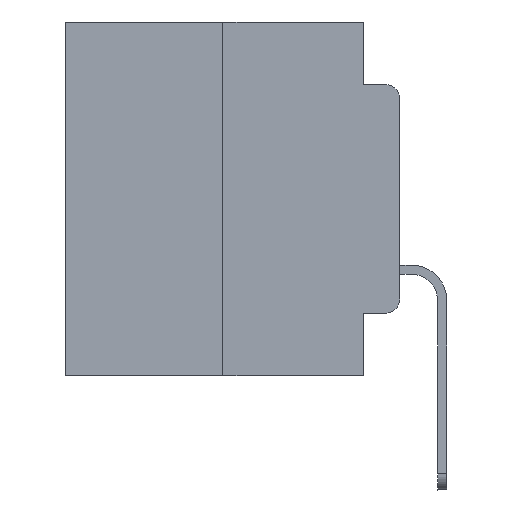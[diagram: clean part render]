
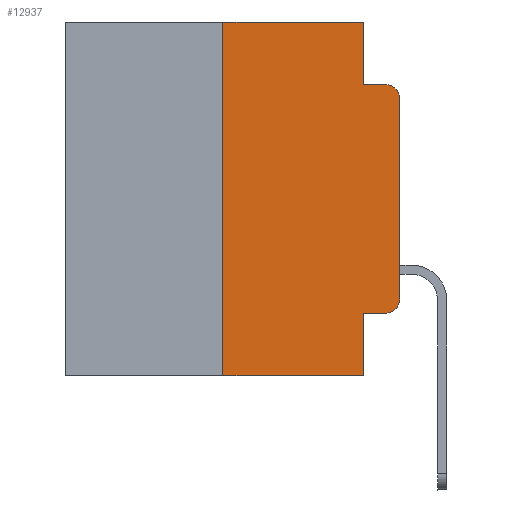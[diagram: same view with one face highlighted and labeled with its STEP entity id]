
A CAD part, left-side view. The second image highlights one B-rep face of the part: STEP entity #12937.
In plain terms, the highlighted planar face has unit normal (-1, 0, 0).
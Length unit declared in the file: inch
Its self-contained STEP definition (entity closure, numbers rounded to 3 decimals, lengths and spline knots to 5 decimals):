
#37 = VERTEX_POINT ( 'NONE', #889 ) ;
#81 = VERTEX_POINT ( 'NONE', #19235 ) ;
#333 = CIRCLE ( 'NONE', #19861, 0.02 ) ;
#505 = AXIS2_PLACEMENT_3D ( 'NONE', #17431, #948, #13442 ) ;
#548 = ORIENTED_EDGE ( 'NONE', *, *, #4891, .T. ) ;
#727 = LINE ( 'NONE', #10863, #883 ) ;
#883 = VECTOR ( 'NONE', #7252, 39.37008 ) ;
#889 = CARTESIAN_POINT ( 'NONE',  ( 0., 0.25, -0.5 ) ) ;
#948 = DIRECTION ( 'NONE',  ( 1., 0., 0. ) ) ;
#1350 = CARTESIAN_POINT ( 'NONE',  ( 0., 0.051, -0.4115 ) ) ;
#1603 = VERTEX_POINT ( 'NONE', #5656 ) ;
#1618 = VERTEX_POINT ( 'NONE', #5376 ) ;
#2019 = VECTOR ( 'NONE', #16478, 39.37008 ) ;
#3756 = VERTEX_POINT ( 'NONE', #25233 ) ;
#3914 = EDGE_LOOP ( 'NONE', ( #16381, #23567, #5466, #25305, #15604, #6276, #548, #19834, #11335, #19244 ) ) ;
#4144 = EDGE_CURVE ( 'NONE', #81, #17900, #727, .T. ) ;
#4157 = CARTESIAN_POINT ( 'NONE',  ( 0., 0.051, 0. ) ) ;
#4180 = VERTEX_POINT ( 'NONE', #17103 ) ;
#4891 = EDGE_CURVE ( 'NONE', #37, #17900, #12891, .T. ) ;
#5034 = CARTESIAN_POINT ( 'NONE',  ( 0., 0.02, -0.1085 ) ) ;
#5376 = CARTESIAN_POINT ( 'NONE',  ( 0., 0.02, -0.0885 ) ) ;
#5466 = ORIENTED_EDGE ( 'NONE', *, *, #22309, .F. ) ;
#5656 = CARTESIAN_POINT ( 'NONE',  ( 0., 0., -0.1085 ) ) ;
#6098 = LINE ( 'NONE', #6337, #12428 ) ;
#6172 = LINE ( 'NONE', #4157, #25601 ) ;
#6267 = CARTESIAN_POINT ( 'NONE',  ( 0., 0.051, 0. ) ) ;
#6276 = ORIENTED_EDGE ( 'NONE', *, *, #20710, .F. ) ;
#6282 = AXIS2_PLACEMENT_3D ( 'NONE', #9366, #13472, #17469 ) ;
#6337 = CARTESIAN_POINT ( 'NONE',  ( 0., 0., 0. ) ) ;
#6486 = CARTESIAN_POINT ( 'NONE',  ( 0., 0., -0.3915 ) ) ;
#7252 = DIRECTION ( 'NONE',  ( 0., 0., -1. ) ) ;
#7475 = CARTESIAN_POINT ( 'NONE',  ( 0., 0.051, -0.5 ) ) ;
#8793 = CARTESIAN_POINT ( 'NONE',  ( 0., 0.051, -0.0885 ) ) ;
#8844 = CIRCLE ( 'NONE', #6282, 0.02 ) ;
#8915 = DIRECTION ( 'NONE',  ( 0., 0., -1. ) ) ;
#9297 = DIRECTION ( 'NONE',  ( 0., -1., 0. ) ) ;
#9366 = CARTESIAN_POINT ( 'NONE',  ( 0., 0.02, -0.3915 ) ) ;
#9746 = LINE ( 'NONE', #1350, #24771 ) ;
#10002 = VERTEX_POINT ( 'NONE', #8793 ) ;
#10120 = CARTESIAN_POINT ( 'NONE',  ( 0., 0.473, 0. ) ) ;
#10453 = VERTEX_POINT ( 'NONE', #6486 ) ;
#10511 = CARTESIAN_POINT ( 'NONE',  ( 0., 0.051, -0.0885 ) ) ;
#10863 = CARTESIAN_POINT ( 'NONE',  ( 0., 0.051, 0. ) ) ;
#11335 = ORIENTED_EDGE ( 'NONE', *, *, #19084, .T. ) ;
#12288 = DIRECTION ( 'NONE',  ( 0., 0., -1. ) ) ;
#12428 = VECTOR ( 'NONE', #20310, 39.37008 ) ;
#12651 = CARTESIAN_POINT ( 'NONE',  ( 0., 0.25, 0. ) ) ;
#12891 = LINE ( 'NONE', #16866, #25067 ) ;
#12937 = ADVANCED_FACE ( 'NONE', ( #19157 ), #17044, .F. ) ;
#13017 = DIRECTION ( 'NONE',  ( 0., -1., 0. ) ) ;
#13349 = EDGE_CURVE ( 'NONE', #3756, #19310, #14244, .T. ) ;
#13442 = DIRECTION ( 'NONE',  ( 0., 0., -1. ) ) ;
#13472 = DIRECTION ( 'NONE',  ( -1., 0., 0. ) ) ;
#13610 = EDGE_CURVE ( 'NONE', #10453, #1603, #6098, .T. ) ;
#14244 = LINE ( 'NONE', #10120, #24319 ) ;
#14882 = DIRECTION ( 'NONE',  ( -1., 0., 0. ) ) ;
#15604 = ORIENTED_EDGE ( 'NONE', *, *, #13349, .F. ) ;
#16381 = ORIENTED_EDGE ( 'NONE', *, *, #13610, .T. ) ;
#16478 = DIRECTION ( 'NONE',  ( 0., -1., 0. ) ) ;
#16866 = CARTESIAN_POINT ( 'NONE',  ( 0., 0.473, -0.5 ) ) ;
#17039 = LINE ( 'NONE', #12651, #23143 ) ;
#17044 = PLANE ( 'NONE',  #505 ) ;
#17103 = CARTESIAN_POINT ( 'NONE',  ( 0., 0.02, -0.4115 ) ) ;
#17431 = CARTESIAN_POINT ( 'NONE',  ( 0., 0.473, 0. ) ) ;
#17469 = DIRECTION ( 'NONE',  ( 0., 0., -1. ) ) ;
#17725 = LINE ( 'NONE', #10511, #2019 ) ;
#17900 = VERTEX_POINT ( 'NONE', #7475 ) ;
#18891 = DIRECTION ( 'NONE',  ( 0., 0., 1. ) ) ;
#18921 = EDGE_CURVE ( 'NONE', #19310, #10002, #6172, .T. ) ;
#19084 = EDGE_CURVE ( 'NONE', #81, #4180, #9746, .T. ) ;
#19157 = FACE_OUTER_BOUND ( 'NONE', #3914, .T. ) ;
#19235 = CARTESIAN_POINT ( 'NONE',  ( 0., 0.051, -0.4115 ) ) ;
#19244 = ORIENTED_EDGE ( 'NONE', *, *, #22171, .T. ) ;
#19310 = VERTEX_POINT ( 'NONE', #6267 ) ;
#19834 = ORIENTED_EDGE ( 'NONE', *, *, #4144, .F. ) ;
#19861 = AXIS2_PLACEMENT_3D ( 'NONE', #5034, #14882, #8915 ) ;
#20310 = DIRECTION ( 'NONE',  ( 0., 0., 1. ) ) ;
#20710 = EDGE_CURVE ( 'NONE', #37, #3756, #17039, .T. ) ;
#22171 = EDGE_CURVE ( 'NONE', #4180, #10453, #8844, .T. ) ;
#22309 = EDGE_CURVE ( 'NONE', #10002, #1618, #17725, .T. ) ;
#22513 = EDGE_CURVE ( 'NONE', #1603, #1618, #333, .T. ) ;
#23143 = VECTOR ( 'NONE', #18891, 39.37008 ) ;
#23567 = ORIENTED_EDGE ( 'NONE', *, *, #22513, .T. ) ;
#23826 = DIRECTION ( 'NONE',  ( 0., -1., 0. ) ) ;
#24319 = VECTOR ( 'NONE', #9297, 39.37008 ) ;
#24771 = VECTOR ( 'NONE', #23826, 39.37008 ) ;
#25067 = VECTOR ( 'NONE', #13017, 39.37008 ) ;
#25233 = CARTESIAN_POINT ( 'NONE',  ( 0., 0.25, 0. ) ) ;
#25305 = ORIENTED_EDGE ( 'NONE', *, *, #18921, .F. ) ;
#25601 = VECTOR ( 'NONE', #12288, 39.37008 ) ;
